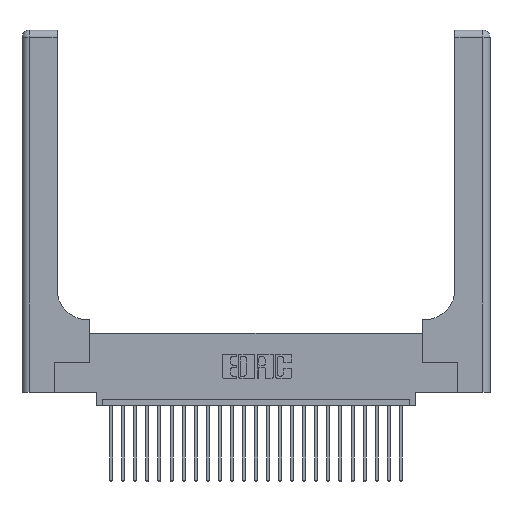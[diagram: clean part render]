
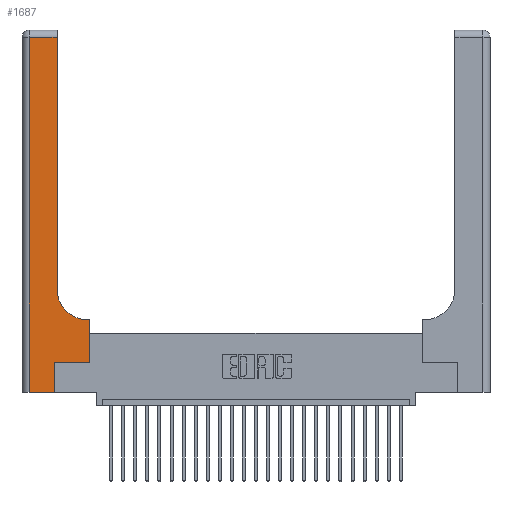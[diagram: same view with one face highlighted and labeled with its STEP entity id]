
A CAD part, top view. The second image highlights one B-rep face of the part: STEP entity #1687.
In plain terms, the highlighted planar face has unit normal (0, 0, 1).
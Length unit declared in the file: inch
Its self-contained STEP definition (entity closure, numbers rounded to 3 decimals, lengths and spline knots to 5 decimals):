
#163 = DIRECTION ( 'NONE',  ( -1., 0., 0. ) ) ;
#515 = DIRECTION ( 'NONE',  ( -1., 0., 0. ) ) ;
#563 = DIRECTION ( 'NONE',  ( 1., 0., 0. ) ) ;
#1687 = ADVANCED_FACE ( 'NONE', ( #15675 ), #19007, .F. ) ;
#1774 = LINE ( 'NONE', #20328, #12625 ) ;
#1784 = CARTESIAN_POINT ( 'NONE',  ( 0.269, 0., 0.37 ) ) ;
#1825 = AXIS2_PLACEMENT_3D ( 'NONE', #8689, #17063, #515 ) ;
#2344 = DIRECTION ( 'NONE',  ( 1., 0., 0. ) ) ;
#2739 = VERTEX_POINT ( 'NONE', #15260 ) ;
#3863 = EDGE_CURVE ( 'NONE', #7498, #6500, #12117, .T. ) ;
#4252 = DIRECTION ( 'NONE',  ( 0., 1., 0. ) ) ;
#4441 = ORIENTED_EDGE ( 'NONE', *, *, #21417, .T. ) ;
#4894 = CARTESIAN_POINT ( 'NONE',  ( 0.5415, 0.85, 0.37 ) ) ;
#5193 = LINE ( 'NONE', #26126, #8079 ) ;
#6240 = ORIENTED_EDGE ( 'NONE', *, *, #14989, .T. ) ;
#6500 = VERTEX_POINT ( 'NONE', #1784 ) ;
#6958 = ORIENTED_EDGE ( 'NONE', *, *, #24860, .T. ) ;
#7498 = VERTEX_POINT ( 'NONE', #9752 ) ;
#8001 = DIRECTION ( 'NONE',  ( 1., 0., 0. ) ) ;
#8079 = VECTOR ( 'NONE', #8001, 39.37008 ) ;
#8689 = CARTESIAN_POINT ( 'NONE',  ( 0., 3., 0.37 ) ) ;
#8890 = CARTESIAN_POINT ( 'NONE',  ( 0.5415, 0.6, 0.37 ) ) ;
#9046 = VECTOR ( 'NONE', #10851, 39.37008 ) ;
#9731 = EDGE_LOOP ( 'NONE', ( #26324, #6958, #21529, #12953, #17590, #21512, #25503, #6240, #4441 ) ) ;
#9752 = CARTESIAN_POINT ( 'NONE',  ( 0.06, 0., 0.37 ) ) ;
#10308 = EDGE_CURVE ( 'NONE', #20865, #7498, #19855, .T. ) ;
#10382 = CARTESIAN_POINT ( 'NONE',  ( 0., 0., 0.37 ) ) ;
#10851 = DIRECTION ( 'NONE',  ( 0., -1., 0. ) ) ;
#10872 = VECTOR ( 'NONE', #4252, 39.37008 ) ;
#11188 = LINE ( 'NONE', #14389, #10872 ) ;
#12117 = LINE ( 'NONE', #10382, #18478 ) ;
#12312 = VERTEX_POINT ( 'NONE', #18306 ) ;
#12625 = VECTOR ( 'NONE', #163, 39.37008 ) ;
#12953 = ORIENTED_EDGE ( 'NONE', *, *, #3863, .T. ) ;
#12972 = CARTESIAN_POINT ( 'NONE',  ( 0.06, 3., 0.37 ) ) ;
#13225 = VECTOR ( 'NONE', #17969, 39.37008 ) ;
#13451 = VERTEX_POINT ( 'NONE', #8890 ) ;
#13918 = EDGE_CURVE ( 'NONE', #16045, #17082, #5193, .T. ) ;
#14389 = CARTESIAN_POINT ( 'NONE',  ( 0.5585, 0.25, 0.37 ) ) ;
#14732 = EDGE_CURVE ( 'NONE', #17082, #23505, #11188, .T. ) ;
#14989 = EDGE_CURVE ( 'NONE', #23505, #13451, #17565, .T. ) ;
#15050 = LINE ( 'NONE', #20393, #18249 ) ;
#15260 = CARTESIAN_POINT ( 'NONE',  ( 0.2915, 0.85, 0.37 ) ) ;
#15411 = CARTESIAN_POINT ( 'NONE',  ( 0.5585, 0.6, 0.37 ) ) ;
#15465 = CARTESIAN_POINT ( 'NONE',  ( 0.5585, 0.25, 0.37 ) ) ;
#15675 = FACE_OUTER_BOUND ( 'NONE', #9731, .T. ) ;
#15897 = AXIS2_PLACEMENT_3D ( 'NONE', #4894, #25090, #563 ) ;
#16045 = VERTEX_POINT ( 'NONE', #19918 ) ;
#17063 = DIRECTION ( 'NONE',  ( 0., 0., -1. ) ) ;
#17082 = VERTEX_POINT ( 'NONE', #15465 ) ;
#17565 = LINE ( 'NONE', #17579, #25495 ) ;
#17579 = CARTESIAN_POINT ( 'NONE',  ( 0.2915, 0.6, 0.37 ) ) ;
#17590 = ORIENTED_EDGE ( 'NONE', *, *, #17803, .T. ) ;
#17803 = EDGE_CURVE ( 'NONE', #6500, #16045, #25634, .T. ) ;
#17969 = DIRECTION ( 'NONE',  ( 0., 1., 0. ) ) ;
#18249 = VECTOR ( 'NONE', #20473, 39.37008 ) ;
#18306 = CARTESIAN_POINT ( 'NONE',  ( 0.2915, 2.94, 0.37 ) ) ;
#18478 = VECTOR ( 'NONE', #2344, 39.37008 ) ;
#19007 = PLANE ( 'NONE',  #1825 ) ;
#19855 = LINE ( 'NONE', #12972, #9046 ) ;
#19918 = CARTESIAN_POINT ( 'NONE',  ( 0.269, 0.25, 0.37 ) ) ;
#19927 = CARTESIAN_POINT ( 'NONE',  ( 0.269, 0., 0.37 ) ) ;
#20328 = CARTESIAN_POINT ( 'NONE',  ( 0., 2.94, 0.37 ) ) ;
#20393 = CARTESIAN_POINT ( 'NONE',  ( 0.2915, 3., 0.37 ) ) ;
#20473 = DIRECTION ( 'NONE',  ( 0., 1., 0. ) ) ;
#20651 = CARTESIAN_POINT ( 'NONE',  ( 0.06, 2.94, 0.37 ) ) ;
#20782 = EDGE_CURVE ( 'NONE', #2739, #12312, #15050, .T. ) ;
#20865 = VERTEX_POINT ( 'NONE', #20651 ) ;
#21392 = CIRCLE ( 'NONE', #15897, 0.25 ) ;
#21417 = EDGE_CURVE ( 'NONE', #13451, #2739, #21392, .T. ) ;
#21512 = ORIENTED_EDGE ( 'NONE', *, *, #13918, .T. ) ;
#21529 = ORIENTED_EDGE ( 'NONE', *, *, #10308, .T. ) ;
#23505 = VERTEX_POINT ( 'NONE', #15411 ) ;
#23710 = DIRECTION ( 'NONE',  ( -1., 0., 0. ) ) ;
#24860 = EDGE_CURVE ( 'NONE', #12312, #20865, #1774, .T. ) ;
#25090 = DIRECTION ( 'NONE',  ( 0., 0., -1. ) ) ;
#25495 = VECTOR ( 'NONE', #23710, 39.37008 ) ;
#25503 = ORIENTED_EDGE ( 'NONE', *, *, #14732, .T. ) ;
#25634 = LINE ( 'NONE', #19927, #13225 ) ;
#26126 = CARTESIAN_POINT ( 'NONE',  ( 0.269, 0.25, 0.37 ) ) ;
#26324 = ORIENTED_EDGE ( 'NONE', *, *, #20782, .T. ) ;
